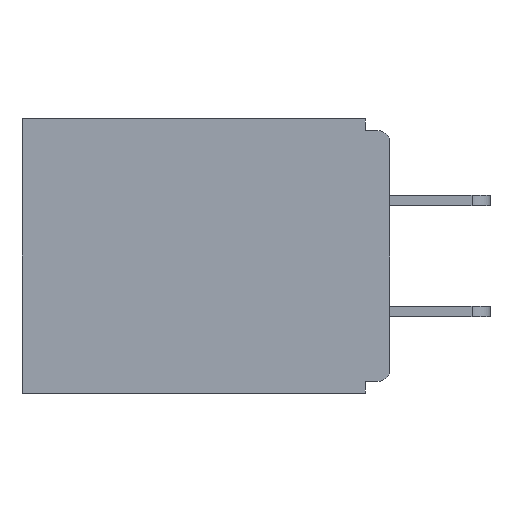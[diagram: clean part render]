
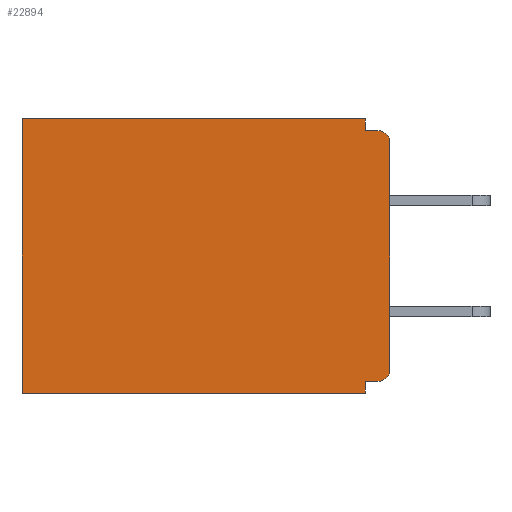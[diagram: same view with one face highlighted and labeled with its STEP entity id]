
A CAD part, left-side view. The second image highlights one B-rep face of the part: STEP entity #22894.
In plain terms, the highlighted planar face has unit normal (-1, 0, 0).
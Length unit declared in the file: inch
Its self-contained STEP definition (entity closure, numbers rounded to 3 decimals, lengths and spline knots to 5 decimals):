
#194 = AXIS2_PLACEMENT_3D ( 'NONE', #17145, #12895, #19410 ) ;
#318 = CIRCLE ( 'NONE', #194, 0.015 ) ;
#382 = DIRECTION ( 'NONE',  ( 0., 0., -1. ) ) ;
#675 = PLANE ( 'NONE',  #12892 ) ;
#740 = AXIS2_PLACEMENT_3D ( 'NONE', #20261, #2486, #7003 ) ;
#1858 = VECTOR ( 'NONE', #11646, 39.37008 ) ;
#2486 = DIRECTION ( 'NONE',  ( -1., 0., 0. ) ) ;
#2889 = DIRECTION ( 'NONE',  ( 1., 0., 0. ) ) ;
#2956 = ORIENTED_EDGE ( 'NONE', *, *, #3086, .F. ) ;
#3086 = EDGE_CURVE ( 'NONE', #12407, #12150, #27510, .T. ) ;
#3255 = CARTESIAN_POINT ( 'NONE',  ( 0.298, 0., -0.343 ) ) ;
#3624 = DIRECTION ( 'NONE',  ( 0., -1., 0. ) ) ;
#3913 = EDGE_CURVE ( 'NONE', #21957, #26492, #28488, .T. ) ;
#4228 = CARTESIAN_POINT ( 'NONE',  ( 0.298, 0.031, -0.343 ) ) ;
#4230 = LINE ( 'NONE', #4883, #1858 ) ;
#4400 = FACE_OUTER_BOUND ( 'NONE', #17633, .T. ) ;
#4606 = ORIENTED_EDGE ( 'NONE', *, *, #27215, .F. ) ;
#4883 = CARTESIAN_POINT ( 'NONE',  ( 0.298, 0., -0.328 ) ) ;
#4960 = CARTESIAN_POINT ( 'NONE',  ( 0.298, 0.031, 0. ) ) ;
#4992 = ORIENTED_EDGE ( 'NONE', *, *, #17454, .F. ) ;
#5016 = CARTESIAN_POINT ( 'NONE',  ( 0.298, 0.015, -0.015 ) ) ;
#5378 = ORIENTED_EDGE ( 'NONE', *, *, #22955, .T. ) ;
#6005 = LINE ( 'NONE', #7369, #26124 ) ;
#7003 = DIRECTION ( 'NONE',  ( 0., 0., -1. ) ) ;
#7164 = VERTEX_POINT ( 'NONE', #4960 ) ;
#7229 = LINE ( 'NONE', #21627, #7591 ) ;
#7369 = CARTESIAN_POINT ( 'NONE',  ( 0.298, 0., 0. ) ) ;
#7591 = VECTOR ( 'NONE', #8421, 39.37008 ) ;
#7847 = CARTESIAN_POINT ( 'NONE',  ( 0.298, 0., -0.015 ) ) ;
#8213 = CARTESIAN_POINT ( 'NONE',  ( 0.298, 0.015, -0.328 ) ) ;
#8300 = CARTESIAN_POINT ( 'NONE',  ( 0.298, 0.46, -0.343 ) ) ;
#8396 = ORIENTED_EDGE ( 'NONE', *, *, #28335, .T. ) ;
#8421 = DIRECTION ( 'NONE',  ( 0., 0., -1. ) ) ;
#8544 = VECTOR ( 'NONE', #8545, 39.37008 ) ;
#8545 = DIRECTION ( 'NONE',  ( 0., 1., 0. ) ) ;
#9193 = VERTEX_POINT ( 'NONE', #25089 ) ;
#9559 = DIRECTION ( 'NONE',  ( 0., 0., -1. ) ) ;
#9933 = LINE ( 'NONE', #17363, #8544 ) ;
#11084 = CARTESIAN_POINT ( 'NONE',  ( 0.298, 0.46, 0. ) ) ;
#11646 = DIRECTION ( 'NONE',  ( 0., 1., 0. ) ) ;
#12150 = VERTEX_POINT ( 'NONE', #8300 ) ;
#12371 = VECTOR ( 'NONE', #17934, 39.37008 ) ;
#12407 = VERTEX_POINT ( 'NONE', #4228 ) ;
#12623 = VERTEX_POINT ( 'NONE', #16187 ) ;
#12892 = AXIS2_PLACEMENT_3D ( 'NONE', #16109, #2889, #13972 ) ;
#12895 = DIRECTION ( 'NONE',  ( -1., 0., 0. ) ) ;
#13448 = CARTESIAN_POINT ( 'NONE',  ( 0.298, 0.031, -0.015 ) ) ;
#13639 = ORIENTED_EDGE ( 'NONE', *, *, #22989, .F. ) ;
#13731 = LINE ( 'NONE', #22515, #12371 ) ;
#13972 = DIRECTION ( 'NONE',  ( 0., 0., -1. ) ) ;
#14316 = VECTOR ( 'NONE', #382, 39.37008 ) ;
#15027 = CARTESIAN_POINT ( 'NONE',  ( 0.298, 0.46, 0. ) ) ;
#15976 = VECTOR ( 'NONE', #3624, 39.37008 ) ;
#16109 = CARTESIAN_POINT ( 'NONE',  ( 0.298, 0., 0. ) ) ;
#16187 = CARTESIAN_POINT ( 'NONE',  ( 0.298, 0., -0.313 ) ) ;
#16527 = EDGE_CURVE ( 'NONE', #17125, #12150, #26845, .T. ) ;
#17125 = VERTEX_POINT ( 'NONE', #15027 ) ;
#17145 = CARTESIAN_POINT ( 'NONE',  ( 0.298, 0.015, -0.313 ) ) ;
#17363 = CARTESIAN_POINT ( 'NONE',  ( 0.298, 0., 0. ) ) ;
#17454 = EDGE_CURVE ( 'NONE', #21930, #26492, #27847, .T. ) ;
#17597 = EDGE_CURVE ( 'NONE', #23769, #9193, #4230, .T. ) ;
#17633 = EDGE_LOOP ( 'NONE', ( #19358, #4992, #4606, #5378, #18279, #2956, #13639, #23766, #8396, #28682 ) ) ;
#17934 = DIRECTION ( 'NONE',  ( 0., 0., -1. ) ) ;
#18279 = ORIENTED_EDGE ( 'NONE', *, *, #16527, .T. ) ;
#19132 = VECTOR ( 'NONE', #22994, 39.37008 ) ;
#19358 = ORIENTED_EDGE ( 'NONE', *, *, #3913, .T. ) ;
#19410 = DIRECTION ( 'NONE',  ( 0., 0., -1. ) ) ;
#20055 = CARTESIAN_POINT ( 'NONE',  ( 0.298, 0., -0.03 ) ) ;
#20261 = CARTESIAN_POINT ( 'NONE',  ( 0.298, 0.015, -0.03 ) ) ;
#21627 = CARTESIAN_POINT ( 'NONE',  ( 0.298, 0.031, -0.343 ) ) ;
#21930 = VERTEX_POINT ( 'NONE', #13448 ) ;
#21957 = VERTEX_POINT ( 'NONE', #20055 ) ;
#22515 = CARTESIAN_POINT ( 'NONE',  ( 0.298, 0.031, -0.343 ) ) ;
#22894 = ADVANCED_FACE ( 'NONE', ( #4400 ), #675, .F. ) ;
#22955 = EDGE_CURVE ( 'NONE', #7164, #17125, #9933, .T. ) ;
#22989 = EDGE_CURVE ( 'NONE', #9193, #12407, #13731, .T. ) ;
#22994 = DIRECTION ( 'NONE',  ( 0., 1., 0. ) ) ;
#23766 = ORIENTED_EDGE ( 'NONE', *, *, #17597, .F. ) ;
#23769 = VERTEX_POINT ( 'NONE', #8213 ) ;
#25089 = CARTESIAN_POINT ( 'NONE',  ( 0.298, 0.031, -0.328 ) ) ;
#25521 = EDGE_CURVE ( 'NONE', #21957, #12623, #6005, .T. ) ;
#26124 = VECTOR ( 'NONE', #9559, 39.37008 ) ;
#26492 = VERTEX_POINT ( 'NONE', #5016 ) ;
#26845 = LINE ( 'NONE', #11084, #14316 ) ;
#27215 = EDGE_CURVE ( 'NONE', #7164, #21930, #7229, .T. ) ;
#27510 = LINE ( 'NONE', #3255, #19132 ) ;
#27847 = LINE ( 'NONE', #7847, #15976 ) ;
#28335 = EDGE_CURVE ( 'NONE', #23769, #12623, #318, .T. ) ;
#28488 = CIRCLE ( 'NONE', #740, 0.015 ) ;
#28682 = ORIENTED_EDGE ( 'NONE', *, *, #25521, .F. ) ;
